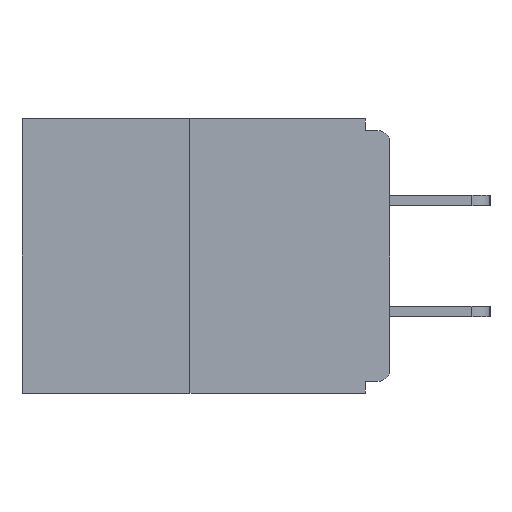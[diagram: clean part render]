
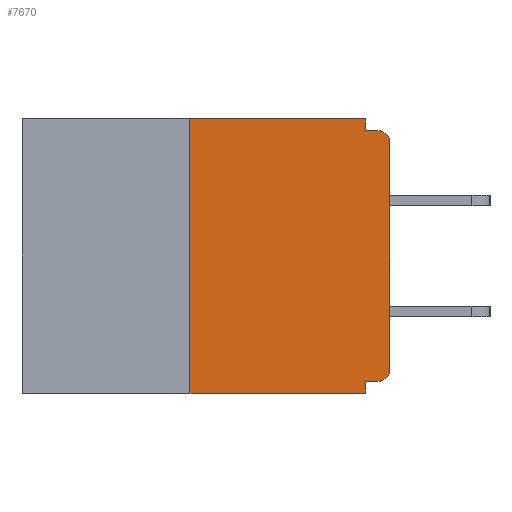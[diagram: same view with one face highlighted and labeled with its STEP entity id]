
A CAD part, left-side view. The second image highlights one B-rep face of the part: STEP entity #7670.
In plain terms, the highlighted planar face has unit normal (-1, 0, 0).
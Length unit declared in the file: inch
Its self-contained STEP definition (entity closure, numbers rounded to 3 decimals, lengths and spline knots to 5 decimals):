
#152 = CARTESIAN_POINT ( 'NONE',  ( 0., 0., -0.328 ) ) ;
#277 = CARTESIAN_POINT ( 'NONE',  ( 0., 0., -0.03 ) ) ;
#745 = DIRECTION ( 'NONE',  ( 0., 0., -1. ) ) ;
#1790 = VERTEX_POINT ( 'NONE', #26119 ) ;
#1862 = CARTESIAN_POINT ( 'NONE',  ( 0., 0.015, -0.015 ) ) ;
#2002 = DIRECTION ( 'NONE',  ( 0., -1., 0. ) ) ;
#3242 = CARTESIAN_POINT ( 'NONE',  ( 0., 0.031, 0. ) ) ;
#3300 = CARTESIAN_POINT ( 'NONE',  ( 0., 0.031, -0.343 ) ) ;
#3328 = CARTESIAN_POINT ( 'NONE',  ( 0., 0.25, -0.343 ) ) ;
#3420 = VECTOR ( 'NONE', #2002, 39.37008 ) ;
#3553 = ORIENTED_EDGE ( 'NONE', *, *, #18713, .F. ) ;
#3575 = DIRECTION ( 'NONE',  ( 0., 0., -1. ) ) ;
#3987 = ORIENTED_EDGE ( 'NONE', *, *, #15967, .T. ) ;
#4171 = EDGE_CURVE ( 'NONE', #15337, #22956, #18499, .T. ) ;
#4652 = LINE ( 'NONE', #3242, #17123 ) ;
#4683 = VERTEX_POINT ( 'NONE', #1862 ) ;
#4890 = CARTESIAN_POINT ( 'NONE',  ( 0., 0.25, 0. ) ) ;
#5137 = ORIENTED_EDGE ( 'NONE', *, *, #7020, .T. ) ;
#5421 = CIRCLE ( 'NONE', #10700, 0.015 ) ;
#5572 = CARTESIAN_POINT ( 'NONE',  ( 0., 0., 0. ) ) ;
#6203 = DIRECTION ( 'NONE',  ( 0., -1., 0. ) ) ;
#6520 = VECTOR ( 'NONE', #19937, 39.37008 ) ;
#6690 = ORIENTED_EDGE ( 'NONE', *, *, #17458, .F. ) ;
#6899 = DIRECTION ( 'NONE',  ( 1., 0., 0. ) ) ;
#7020 = EDGE_CURVE ( 'NONE', #11913, #27081, #22799, .T. ) ;
#7076 = CARTESIAN_POINT ( 'NONE',  ( 0., 0.46, 0. ) ) ;
#7670 = ADVANCED_FACE ( 'NONE', ( #26703 ), #25602, .F. ) ;
#7882 = ORIENTED_EDGE ( 'NONE', *, *, #19022, .F. ) ;
#8057 = EDGE_CURVE ( 'NONE', #20508, #16121, #18504, .T. ) ;
#8966 = DIRECTION ( 'NONE',  ( 0., -1., 0. ) ) ;
#9862 = CARTESIAN_POINT ( 'NONE',  ( 0., 0.015, -0.03 ) ) ;
#9928 = DIRECTION ( 'NONE',  ( 0., 0., 1. ) ) ;
#10210 = DIRECTION ( 'NONE',  ( -1., 0., 0. ) ) ;
#10597 = ORIENTED_EDGE ( 'NONE', *, *, #4171, .F. ) ;
#10700 = AXIS2_PLACEMENT_3D ( 'NONE', #16213, #10210, #18458 ) ;
#10911 = ORIENTED_EDGE ( 'NONE', *, *, #21373, .F. ) ;
#11492 = DIRECTION ( 'NONE',  ( 0., 0., 1. ) ) ;
#11663 = DIRECTION ( 'NONE',  ( 0., 0., -1. ) ) ;
#11913 = VERTEX_POINT ( 'NONE', #15689 ) ;
#12111 = LINE ( 'NONE', #3300, #6520 ) ;
#12476 = CARTESIAN_POINT ( 'NONE',  ( 0., 0.031, -0.343 ) ) ;
#13935 = VECTOR ( 'NONE', #11492, 39.37008 ) ;
#13959 = VECTOR ( 'NONE', #8966, 39.37008 ) ;
#14582 = CARTESIAN_POINT ( 'NONE',  ( 0., 0.46, 0. ) ) ;
#15009 = VECTOR ( 'NONE', #6203, 39.37008 ) ;
#15337 = VERTEX_POINT ( 'NONE', #19395 ) ;
#15689 = CARTESIAN_POINT ( 'NONE',  ( 0., 0., -0.313 ) ) ;
#15967 = EDGE_CURVE ( 'NONE', #15337, #11913, #5421, .T. ) ;
#16121 = VERTEX_POINT ( 'NONE', #12476 ) ;
#16141 = EDGE_CURVE ( 'NONE', #22664, #1790, #18513, .T. ) ;
#16213 = CARTESIAN_POINT ( 'NONE',  ( 0., 0.015, -0.313 ) ) ;
#16923 = ORIENTED_EDGE ( 'NONE', *, *, #8057, .T. ) ;
#17123 = VECTOR ( 'NONE', #11663, 39.37008 ) ;
#17186 = LINE ( 'NONE', #24092, #13935 ) ;
#17458 = EDGE_CURVE ( 'NONE', #1790, #25751, #4652, .T. ) ;
#18458 = DIRECTION ( 'NONE',  ( 0., 0., -1. ) ) ;
#18499 = LINE ( 'NONE', #152, #25687 ) ;
#18504 = LINE ( 'NONE', #25810, #13959 ) ;
#18513 = LINE ( 'NONE', #14582, #3420 ) ;
#18713 = EDGE_CURVE ( 'NONE', #22956, #16121, #12111, .T. ) ;
#19022 = EDGE_CURVE ( 'NONE', #25751, #4683, #21508, .T. ) ;
#19333 = CIRCLE ( 'NONE', #23441, 0.015 ) ;
#19395 = CARTESIAN_POINT ( 'NONE',  ( 0., 0.015, -0.328 ) ) ;
#19937 = DIRECTION ( 'NONE',  ( 0., 0., -1. ) ) ;
#20304 = DIRECTION ( 'NONE',  ( -1., 0., 0. ) ) ;
#20508 = VERTEX_POINT ( 'NONE', #3328 ) ;
#20625 = CARTESIAN_POINT ( 'NONE',  ( 0., 0., -0.015 ) ) ;
#20677 = CARTESIAN_POINT ( 'NONE',  ( 0., 0.031, -0.328 ) ) ;
#21143 = AXIS2_PLACEMENT_3D ( 'NONE', #7076, #6899, #745 ) ;
#21184 = VECTOR ( 'NONE', #9928, 39.37008 ) ;
#21373 = EDGE_CURVE ( 'NONE', #20508, #22664, #17186, .T. ) ;
#21508 = LINE ( 'NONE', #20625, #15009 ) ;
#21595 = DIRECTION ( 'NONE',  ( 0., 1., 0. ) ) ;
#22664 = VERTEX_POINT ( 'NONE', #4890 ) ;
#22799 = LINE ( 'NONE', #5572, #21184 ) ;
#22956 = VERTEX_POINT ( 'NONE', #20677 ) ;
#23441 = AXIS2_PLACEMENT_3D ( 'NONE', #9862, #20304, #3575 ) ;
#23769 = EDGE_LOOP ( 'NONE', ( #27017, #10911, #16923, #3553, #10597, #3987, #5137, #23925, #7882, #6690 ) ) ;
#23925 = ORIENTED_EDGE ( 'NONE', *, *, #25815, .T. ) ;
#23936 = CARTESIAN_POINT ( 'NONE',  ( 0., 0.031, -0.015 ) ) ;
#24092 = CARTESIAN_POINT ( 'NONE',  ( 0., 0.25, 0. ) ) ;
#25602 = PLANE ( 'NONE',  #21143 ) ;
#25687 = VECTOR ( 'NONE', #21595, 39.37008 ) ;
#25751 = VERTEX_POINT ( 'NONE', #23936 ) ;
#25810 = CARTESIAN_POINT ( 'NONE',  ( 0., 0.46, -0.343 ) ) ;
#25815 = EDGE_CURVE ( 'NONE', #27081, #4683, #19333, .T. ) ;
#26119 = CARTESIAN_POINT ( 'NONE',  ( 0., 0.031, 0. ) ) ;
#26703 = FACE_OUTER_BOUND ( 'NONE', #23769, .T. ) ;
#27017 = ORIENTED_EDGE ( 'NONE', *, *, #16141, .F. ) ;
#27081 = VERTEX_POINT ( 'NONE', #277 ) ;
